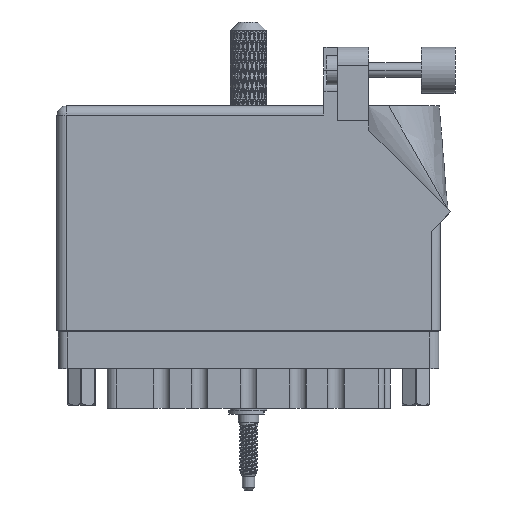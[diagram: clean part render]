
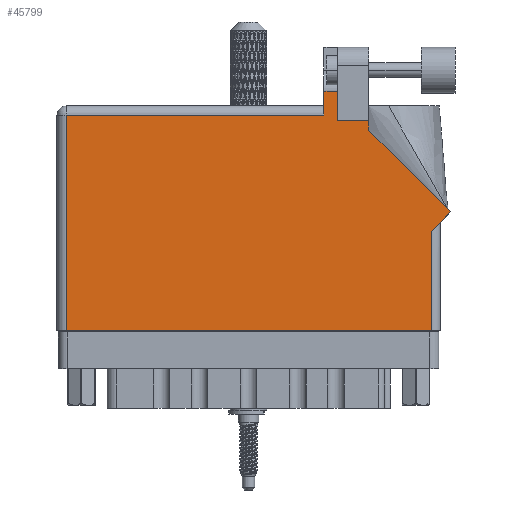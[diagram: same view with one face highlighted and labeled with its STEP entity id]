
A CAD part, front view. The second image highlights one B-rep face of the part: STEP entity #45799.
In plain terms, the highlighted face is planar.
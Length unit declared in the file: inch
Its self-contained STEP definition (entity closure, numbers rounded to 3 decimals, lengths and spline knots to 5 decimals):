
#741 = CARTESIAN_POINT ( 'NONE',  ( 0.062, 0., 0. ) ) ;
#1189 = VECTOR ( 'NONE', #3230, 39.37008 ) ;
#2873 = ORIENTED_EDGE ( 'NONE', *, *, #68783, .T. ) ;
#3230 = DIRECTION ( 'NONE',  ( 0., -1., 0. ) ) ;
#3673 = VERTEX_POINT ( 'NONE', #79778 ) ;
#3799 = VERTEX_POINT ( 'NONE', #32886 ) ;
#6633 = LINE ( 'NONE', #73337, #79980 ) ;
#6994 = AXIS2_PLACEMENT_3D ( 'NONE', #81013, #31647, #71033 ) ;
#8569 = EDGE_CURVE ( 'NONE', #16563, #69285, #13118, .T. ) ;
#9505 = LINE ( 'NONE', #64937, #111146 ) ;
#11480 = EDGE_CURVE ( 'NONE', #43956, #48117, #6633, .T. ) ;
#13118 = LINE ( 'NONE', #113187, #70061 ) ;
#14519 = ORIENTED_EDGE ( 'NONE', *, *, #53296, .T. ) ;
#15148 = LINE ( 'NONE', #109681, #31535 ) ;
#15584 = DIRECTION ( 'NONE',  ( 0.707, 0.707, 0. ) ) ;
#16161 = VERTEX_POINT ( 'NONE', #97758 ) ;
#16563 = VERTEX_POINT ( 'NONE', #40801 ) ;
#17068 = EDGE_CURVE ( 'NONE', #90918, #21337, #123885, .T. ) ;
#17157 = CARTESIAN_POINT ( 'NONE',  ( 1.913, 1.43, 0. ) ) ;
#17592 = LINE ( 'NONE', #117549, #75815 ) ;
#19353 = VERTEX_POINT ( 'NONE', #73578 ) ;
#20465 = EDGE_CURVE ( 'NONE', #3673, #16563, #47190, .T. ) ;
#21337 = VERTEX_POINT ( 'NONE', #60853 ) ;
#22597 = ORIENTED_EDGE ( 'NONE', *, *, #102603, .T. ) ;
#23210 = CARTESIAN_POINT ( 'NONE',  ( 2.126, 1.36442, 0. ) ) ;
#23777 = DIRECTION ( 'NONE',  ( 0., -1., 0. ) ) ;
#25167 = LINE ( 'NONE', #741, #1189 ) ;
#25619 = DIRECTION ( 'NONE',  ( -1., 0., 0. ) ) ;
#29557 = VECTOR ( 'NONE', #50523, 39.37008 ) ;
#31535 = VECTOR ( 'NONE', #112550, 39.37008 ) ;
#31647 = DIRECTION ( 'NONE',  ( 0., 0., -1. ) ) ;
#31653 = CARTESIAN_POINT ( 'NONE',  ( 1.913, 1.43, 0. ) ) ;
#32573 = LINE ( 'NONE', #31653, #29557 ) ;
#32886 = CARTESIAN_POINT ( 'NONE',  ( 2.55, 0., 0. ) ) ;
#34392 = CARTESIAN_POINT ( 'NONE',  ( 2.612, 0.737, 0. ) ) ;
#35159 = EDGE_CURVE ( 'NONE', #19353, #3673, #9505, .T. ) ;
#38602 = EDGE_CURVE ( 'NONE', #84552, #43956, #15148, .T. ) ;
#39869 = ORIENTED_EDGE ( 'NONE', *, *, #11480, .T. ) ;
#40399 = DIRECTION ( 'NONE',  ( 0., 1., 0. ) ) ;
#40801 = CARTESIAN_POINT ( 'NONE',  ( 1.819, 1.468, 0. ) ) ;
#41996 = DIRECTION ( 'NONE',  ( 1., 0., 0. ) ) ;
#43956 = VERTEX_POINT ( 'NONE', #46389 ) ;
#44770 = DIRECTION ( 'NONE',  ( -1., 0., 0. ) ) ;
#45799 = ADVANCED_FACE ( 'NONE', ( #123124 ), #51747, .F. ) ;
#46389 = CARTESIAN_POINT ( 'NONE',  ( 2.126, 1.43, 0. ) ) ;
#47190 = LINE ( 'NONE', #99790, #84610 ) ;
#48117 = VERTEX_POINT ( 'NONE', #17157 ) ;
#49336 = ORIENTED_EDGE ( 'NONE', *, *, #35159, .T. ) ;
#50523 = DIRECTION ( 'NONE',  ( 0., 1., 0. ) ) ;
#51747 = PLANE ( 'NONE',  #6994 ) ;
#51794 = LINE ( 'NONE', #72555, #95136 ) ;
#52440 = DIRECTION ( 'NONE',  ( -0.707, 0.707, 0. ) ) ;
#53296 = EDGE_CURVE ( 'NONE', #48117, #19353, #32573, .T. ) ;
#58061 = EDGE_CURVE ( 'NONE', #69285, #16161, #25167, .T. ) ;
#60342 = ORIENTED_EDGE ( 'NONE', *, *, #8569, .T. ) ;
#60853 = CARTESIAN_POINT ( 'NONE',  ( 2.68271, 0.80771, 0. ) ) ;
#61992 = LINE ( 'NONE', #88035, #115670 ) ;
#64937 = CARTESIAN_POINT ( 'NONE',  ( 2.24377, 1.6315, 0. ) ) ;
#68783 = EDGE_CURVE ( 'NONE', #3799, #90918, #61992, .T. ) ;
#69285 = VERTEX_POINT ( 'NONE', #97521 ) ;
#70061 = VECTOR ( 'NONE', #44770, 39.37008 ) ;
#71033 = DIRECTION ( 'NONE',  ( -1., 0., 0. ) ) ;
#72517 = ORIENTED_EDGE ( 'NONE', *, *, #38602, .T. ) ;
#72555 = CARTESIAN_POINT ( 'NONE',  ( 2.68271, 0.80771, 0. ) ) ;
#73337 = CARTESIAN_POINT ( 'NONE',  ( 2.126, 1.43, 0. ) ) ;
#73578 = CARTESIAN_POINT ( 'NONE',  ( 1.913, 1.6315, 0. ) ) ;
#74037 = CARTESIAN_POINT ( 'NONE',  ( 2.55, 0.675, 0. ) ) ;
#75815 = VECTOR ( 'NONE', #41996, 39.37008 ) ;
#78796 = EDGE_CURVE ( 'NONE', #16161, #3799, #17592, .T. ) ;
#79778 = CARTESIAN_POINT ( 'NONE',  ( 1.819, 1.6315, 0. ) ) ;
#79980 = VECTOR ( 'NONE', #25619, 39.37008 ) ;
#81013 = CARTESIAN_POINT ( 'NONE',  ( 0., 1.53, 0. ) ) ;
#83698 = DIRECTION ( 'NONE',  ( -1., 0., 0. ) ) ;
#84552 = VERTEX_POINT ( 'NONE', #23210 ) ;
#84610 = VECTOR ( 'NONE', #23777, 39.37008 ) ;
#88035 = CARTESIAN_POINT ( 'NONE',  ( 2.55, 0.737, 0. ) ) ;
#90918 = VERTEX_POINT ( 'NONE', #74037 ) ;
#92455 = ORIENTED_EDGE ( 'NONE', *, *, #17068, .T. ) ;
#95136 = VECTOR ( 'NONE', #52440, 39.37008 ) ;
#97521 = CARTESIAN_POINT ( 'NONE',  ( 0.062, 1.468, 0. ) ) ;
#97758 = CARTESIAN_POINT ( 'NONE',  ( 0.062, 0., 0. ) ) ;
#99790 = CARTESIAN_POINT ( 'NONE',  ( 1.819, 1.53, 0. ) ) ;
#101167 = EDGE_LOOP ( 'NONE', ( #14519, #49336, #118154, #60342, #110355, #104550, #2873, #92455, #22597, #72517, #39869 ) ) ;
#102603 = EDGE_CURVE ( 'NONE', #21337, #84552, #51794, .T. ) ;
#104550 = ORIENTED_EDGE ( 'NONE', *, *, #78796, .T. ) ;
#109681 = CARTESIAN_POINT ( 'NONE',  ( 2.126, 1.36442, 0. ) ) ;
#110355 = ORIENTED_EDGE ( 'NONE', *, *, #58061, .T. ) ;
#110473 = VECTOR ( 'NONE', #15584, 39.37008 ) ;
#111146 = VECTOR ( 'NONE', #83698, 39.37008 ) ;
#112550 = DIRECTION ( 'NONE',  ( 0., 1., 0. ) ) ;
#113187 = CARTESIAN_POINT ( 'NONE',  ( 0., 1.468, 0. ) ) ;
#115670 = VECTOR ( 'NONE', #40399, 39.37008 ) ;
#117549 = CARTESIAN_POINT ( 'NONE',  ( 0., 0., 0. ) ) ;
#118154 = ORIENTED_EDGE ( 'NONE', *, *, #20465, .T. ) ;
#123124 = FACE_OUTER_BOUND ( 'NONE', #101167, .T. ) ;
#123885 = LINE ( 'NONE', #34392, #110473 ) ;
